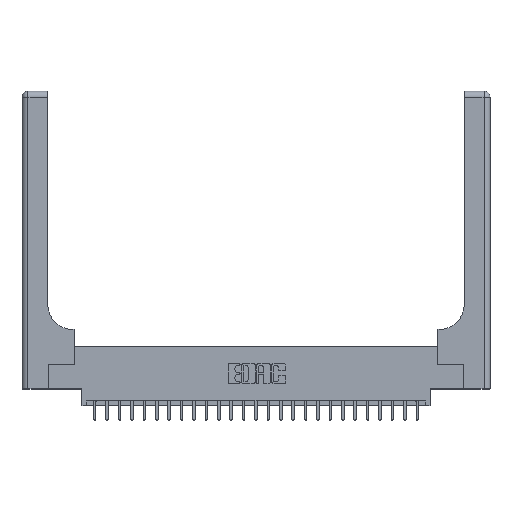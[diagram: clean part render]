
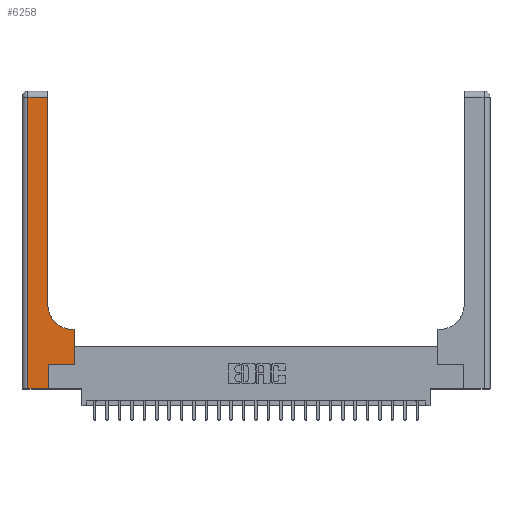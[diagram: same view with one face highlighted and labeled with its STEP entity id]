
A CAD part, top view. The second image highlights one B-rep face of the part: STEP entity #6258.
In plain terms, the highlighted planar face has unit normal (0, 0, 1).
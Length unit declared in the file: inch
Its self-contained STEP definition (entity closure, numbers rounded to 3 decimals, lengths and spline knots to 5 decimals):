
#207 = CARTESIAN_POINT ( 'NONE',  ( 0.51, 0.6, 0.37 ) ) ;
#544 = CARTESIAN_POINT ( 'NONE',  ( 0.26, 0.6, 0.37 ) ) ;
#570 = VECTOR ( 'NONE', #6261, 39.37008 ) ;
#605 = PLANE ( 'NONE',  #21631 ) ;
#613 = ORIENTED_EDGE ( 'NONE', *, *, #3995, .T. ) ;
#781 = VERTEX_POINT ( 'NONE', #6930 ) ;
#1118 = ORIENTED_EDGE ( 'NONE', *, *, #1184, .T. ) ;
#1184 = EDGE_CURVE ( 'NONE', #3403, #18207, #5327, .T. ) ;
#1222 = VECTOR ( 'NONE', #11031, 39.37008 ) ;
#1379 = ORIENTED_EDGE ( 'NONE', *, *, #20283, .T. ) ;
#1416 = VERTEX_POINT ( 'NONE', #18155 ) ;
#2366 = EDGE_CURVE ( 'NONE', #7728, #1416, #8457, .T. ) ;
#3156 = CARTESIAN_POINT ( 'NONE',  ( 0., 2.94, 0.37 ) ) ;
#3160 = DIRECTION ( 'NONE',  ( 1., 0., 0. ) ) ;
#3201 = ORIENTED_EDGE ( 'NONE', *, *, #2366, .T. ) ;
#3403 = VERTEX_POINT ( 'NONE', #207 ) ;
#3471 = CARTESIAN_POINT ( 'NONE',  ( 0.265, 0.25, 0.37 ) ) ;
#3995 = EDGE_CURVE ( 'NONE', #18207, #781, #19185, .T. ) ;
#4135 = LINE ( 'NONE', #544, #20845 ) ;
#5327 = CIRCLE ( 'NONE', #9039, 0.25 ) ;
#5927 = DIRECTION ( 'NONE',  ( 0., 1., 0. ) ) ;
#6258 = ADVANCED_FACE ( 'NONE', ( #18092 ), #605, .F. ) ;
#6261 = DIRECTION ( 'NONE',  ( 0., 1., 0. ) ) ;
#6275 = VECTOR ( 'NONE', #19557, 39.37008 ) ;
#6668 = VERTEX_POINT ( 'NONE', #21755 ) ;
#6827 = DIRECTION ( 'NONE',  ( 0., -1., 0. ) ) ;
#6930 = CARTESIAN_POINT ( 'NONE',  ( 0.26, 2.94, 0.37 ) ) ;
#7728 = VERTEX_POINT ( 'NONE', #11933 ) ;
#8115 = EDGE_LOOP ( 'NONE', ( #613, #25374, #1379, #23157, #10755, #24967, #3201, #19436, #1118 ) ) ;
#8163 = VERTEX_POINT ( 'NONE', #22297 ) ;
#8457 = LINE ( 'NONE', #16174, #570 ) ;
#8886 = VERTEX_POINT ( 'NONE', #9639 ) ;
#9019 = CARTESIAN_POINT ( 'NONE',  ( 0.06, 3., 0.37 ) ) ;
#9039 = AXIS2_PLACEMENT_3D ( 'NONE', #12692, #10909, #3160 ) ;
#9639 = CARTESIAN_POINT ( 'NONE',  ( 0.06, 2.94, 0.37 ) ) ;
#9677 = LINE ( 'NONE', #11367, #6275 ) ;
#10073 = DIRECTION ( 'NONE',  ( -1., 0., 0. ) ) ;
#10127 = DIRECTION ( 'NONE',  ( 0., 0., -1. ) ) ;
#10755 = ORIENTED_EDGE ( 'NONE', *, *, #20877, .T. ) ;
#10909 = DIRECTION ( 'NONE',  ( 0., 0., -1. ) ) ;
#11031 = DIRECTION ( 'NONE',  ( -1., 0., 0. ) ) ;
#11340 = DIRECTION ( 'NONE',  ( 1., 0., 0. ) ) ;
#11367 = CARTESIAN_POINT ( 'NONE',  ( 0., 0., 0.37 ) ) ;
#11933 = CARTESIAN_POINT ( 'NONE',  ( 0.528, 0.25, 0.37 ) ) ;
#12617 = LINE ( 'NONE', #9019, #19854 ) ;
#12692 = CARTESIAN_POINT ( 'NONE',  ( 0.51, 0.85, 0.37 ) ) ;
#13495 = VERTEX_POINT ( 'NONE', #20803 ) ;
#14243 = CARTESIAN_POINT ( 'NONE',  ( 0., 3., 0.37 ) ) ;
#14802 = VECTOR ( 'NONE', #5927, 39.37008 ) ;
#16174 = CARTESIAN_POINT ( 'NONE',  ( 0.528, 0.25, 0.37 ) ) ;
#16292 = DIRECTION ( 'NONE',  ( -1., 0., 0. ) ) ;
#16778 = EDGE_CURVE ( 'NONE', #1416, #3403, #4135, .T. ) ;
#17764 = CARTESIAN_POINT ( 'NONE',  ( 0.26, 3., 0.37 ) ) ;
#18092 = FACE_OUTER_BOUND ( 'NONE', #8115, .T. ) ;
#18155 = CARTESIAN_POINT ( 'NONE',  ( 0.528, 0.6, 0.37 ) ) ;
#18207 = VERTEX_POINT ( 'NONE', #21718 ) ;
#19185 = LINE ( 'NONE', #17764, #14802 ) ;
#19436 = ORIENTED_EDGE ( 'NONE', *, *, #16778, .T. ) ;
#19557 = DIRECTION ( 'NONE',  ( 1., 0., 0. ) ) ;
#19634 = EDGE_CURVE ( 'NONE', #6668, #7728, #21077, .T. ) ;
#19854 = VECTOR ( 'NONE', #6827, 39.37008 ) ;
#20087 = VECTOR ( 'NONE', #20599, 39.37008 ) ;
#20283 = EDGE_CURVE ( 'NONE', #8886, #8163, #12617, .T. ) ;
#20530 = EDGE_CURVE ( 'NONE', #781, #8886, #20760, .T. ) ;
#20599 = DIRECTION ( 'NONE',  ( 0., 1., 0. ) ) ;
#20760 = LINE ( 'NONE', #3156, #1222 ) ;
#20803 = CARTESIAN_POINT ( 'NONE',  ( 0.265, 0., 0.37 ) ) ;
#20845 = VECTOR ( 'NONE', #10073, 39.37008 ) ;
#20877 = EDGE_CURVE ( 'NONE', #13495, #6668, #24615, .T. ) ;
#20986 = CARTESIAN_POINT ( 'NONE',  ( 0.265, 0., 0.37 ) ) ;
#21077 = LINE ( 'NONE', #3471, #23745 ) ;
#21631 = AXIS2_PLACEMENT_3D ( 'NONE', #14243, #10127, #16292 ) ;
#21718 = CARTESIAN_POINT ( 'NONE',  ( 0.26, 0.85, 0.37 ) ) ;
#21755 = CARTESIAN_POINT ( 'NONE',  ( 0.265, 0.25, 0.37 ) ) ;
#22297 = CARTESIAN_POINT ( 'NONE',  ( 0.06, 0., 0.37 ) ) ;
#23157 = ORIENTED_EDGE ( 'NONE', *, *, #25141, .T. ) ;
#23745 = VECTOR ( 'NONE', #11340, 39.37008 ) ;
#24615 = LINE ( 'NONE', #20986, #20087 ) ;
#24967 = ORIENTED_EDGE ( 'NONE', *, *, #19634, .T. ) ;
#25141 = EDGE_CURVE ( 'NONE', #8163, #13495, #9677, .T. ) ;
#25374 = ORIENTED_EDGE ( 'NONE', *, *, #20530, .T. ) ;
